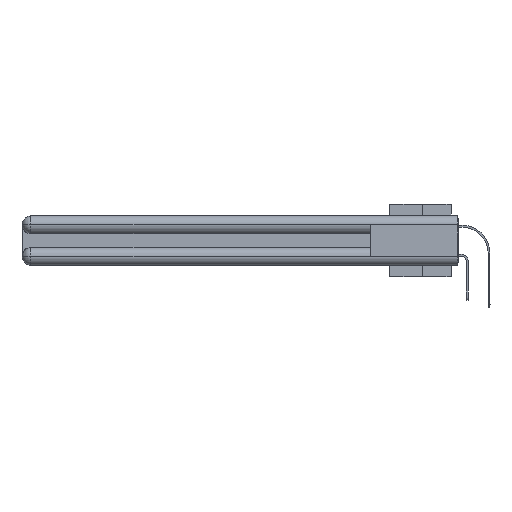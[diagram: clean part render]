
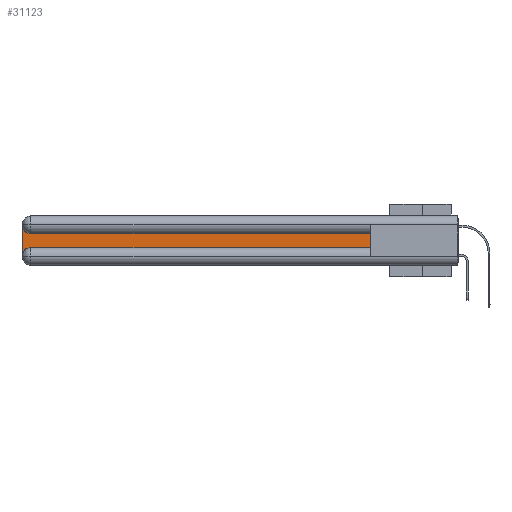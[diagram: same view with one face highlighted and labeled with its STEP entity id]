
A CAD part, left-side view. The second image highlights one B-rep face of the part: STEP entity #31123.
In plain terms, the highlighted planar face has unit normal (-1, 0, 0).
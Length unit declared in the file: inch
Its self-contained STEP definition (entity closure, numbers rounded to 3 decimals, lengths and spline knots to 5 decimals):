
#1071 = LINE ( 'NONE', #18931, #37932 ) ;
#1705 = EDGE_CURVE ( 'NONE', #31615, #38962, #38866, .T. ) ;
#2958 = DIRECTION ( 'NONE',  ( 1., 0., 0. ) ) ;
#4066 = DIRECTION ( 'NONE',  ( 0., 1., 0. ) ) ;
#4200 = VERTEX_POINT ( 'NONE', #18957 ) ;
#5177 = VECTOR ( 'NONE', #10042, 39.37008 ) ;
#8448 = ORIENTED_EDGE ( 'NONE', *, *, #23793, .T. ) ;
#8512 = CARTESIAN_POINT ( 'NONE',  ( 0.075, 3., -0.0625 ) ) ;
#9486 = AXIS2_PLACEMENT_3D ( 'NONE', #11890, #2958, #23982 ) ;
#9853 = LINE ( 'NONE', #37188, #5177 ) ;
#10042 = DIRECTION ( 'NONE',  ( 0., -1., 0. ) ) ;
#10961 = FACE_OUTER_BOUND ( 'NONE', #28610, .T. ) ;
#11890 = CARTESIAN_POINT ( 'NONE',  ( 0.075, 2.94, -0.0625 ) ) ;
#12123 = DIRECTION ( 'NONE',  ( 0., 0., -1. ) ) ;
#12974 = EDGE_CURVE ( 'NONE', #15684, #4200, #9853, .T. ) ;
#13971 = ORIENTED_EDGE ( 'NONE', *, *, #21758, .T. ) ;
#14112 = ORIENTED_EDGE ( 'NONE', *, *, #12974, .T. ) ;
#14139 = CARTESIAN_POINT ( 'NONE',  ( 0.075, 2.94, -0.2775 ) ) ;
#14701 = ORIENTED_EDGE ( 'NONE', *, *, #18003, .T. ) ;
#14890 = CARTESIAN_POINT ( 'NONE',  ( 0.075, 0.6, -0.2175 ) ) ;
#15684 = VERTEX_POINT ( 'NONE', #36444 ) ;
#17211 = AXIS2_PLACEMENT_3D ( 'NONE', #23055, #35122, #35524 ) ;
#17670 = CARTESIAN_POINT ( 'NONE',  ( 0.075, 3., -0.2175 ) ) ;
#18003 = EDGE_CURVE ( 'NONE', #4200, #28983, #38476, .T. ) ;
#18253 = CIRCLE ( 'NONE', #27117, 0.06 ) ;
#18781 = EDGE_CURVE ( 'NONE', #38962, #15684, #18253, .T. ) ;
#18931 = CARTESIAN_POINT ( 'NONE',  ( 0.075, 0.6, -0.1225 ) ) ;
#18957 = CARTESIAN_POINT ( 'NONE',  ( 0.075, 0.6, -0.2175 ) ) ;
#21758 = EDGE_CURVE ( 'NONE', #28983, #29820, #1071, .T. ) ;
#21904 = ORIENTED_EDGE ( 'NONE', *, *, #1705, .T. ) ;
#23055 = CARTESIAN_POINT ( 'NONE',  ( 0.075, 3., -0.1225 ) ) ;
#23793 = EDGE_CURVE ( 'NONE', #29820, #31615, #26590, .T. ) ;
#23982 = DIRECTION ( 'NONE',  ( 0., 0., -1. ) ) ;
#25181 = VECTOR ( 'NONE', #12123, 39.37008 ) ;
#26240 = DIRECTION ( 'NONE',  ( 1., 0., 0. ) ) ;
#26590 = CIRCLE ( 'NONE', #9486, 0.06 ) ;
#27117 = AXIS2_PLACEMENT_3D ( 'NONE', #14139, #26240, #35329 ) ;
#28610 = EDGE_LOOP ( 'NONE', ( #13971, #8448, #21904, #32302, #14112, #14701 ) ) ;
#28983 = VERTEX_POINT ( 'NONE', #32190 ) ;
#29297 = CARTESIAN_POINT ( 'NONE',  ( 0.075, 2.94, -0.1225 ) ) ;
#29820 = VERTEX_POINT ( 'NONE', #29297 ) ;
#31123 = ADVANCED_FACE ( 'NONE', ( #10961 ), #38480, .F. ) ;
#31615 = VERTEX_POINT ( 'NONE', #8512 ) ;
#31666 = CARTESIAN_POINT ( 'NONE',  ( 0.075, 3., -0.2775 ) ) ;
#32190 = CARTESIAN_POINT ( 'NONE',  ( 0.075, 0.6, -0.1225 ) ) ;
#32302 = ORIENTED_EDGE ( 'NONE', *, *, #18781, .T. ) ;
#32760 = VECTOR ( 'NONE', #39056, 39.37008 ) ;
#35122 = DIRECTION ( 'NONE',  ( 1., 0., 0. ) ) ;
#35329 = DIRECTION ( 'NONE',  ( 0., 0., -1. ) ) ;
#35524 = DIRECTION ( 'NONE',  ( 0., 0., -1. ) ) ;
#36444 = CARTESIAN_POINT ( 'NONE',  ( 0.075, 2.94, -0.2175 ) ) ;
#37188 = CARTESIAN_POINT ( 'NONE',  ( 0.075, 0.6, -0.2175 ) ) ;
#37932 = VECTOR ( 'NONE', #4066, 39.37008 ) ;
#38476 = LINE ( 'NONE', #14890, #32760 ) ;
#38480 = PLANE ( 'NONE',  #17211 ) ;
#38866 = LINE ( 'NONE', #17670, #25181 ) ;
#38962 = VERTEX_POINT ( 'NONE', #31666 ) ;
#39056 = DIRECTION ( 'NONE',  ( 0., 0., 1. ) ) ;
